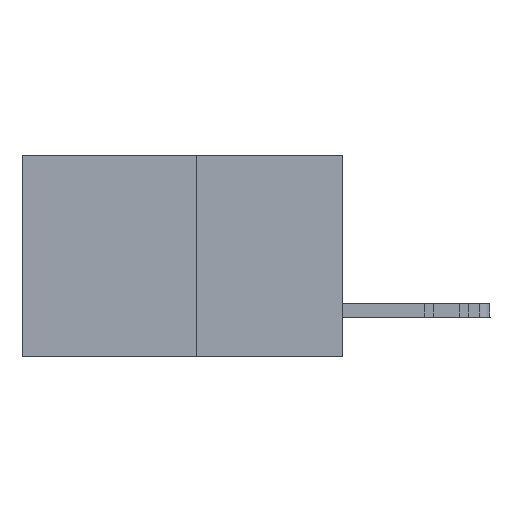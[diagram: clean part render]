
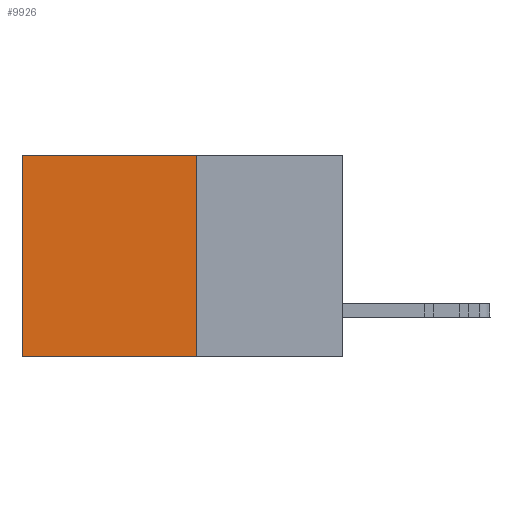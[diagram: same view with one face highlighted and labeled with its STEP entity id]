
A CAD part, left-side view. The second image highlights one B-rep face of the part: STEP entity #9926.
In plain terms, the highlighted planar face has unit normal (-1, 0, 0).
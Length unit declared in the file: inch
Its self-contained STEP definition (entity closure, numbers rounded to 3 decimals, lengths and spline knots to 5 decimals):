
#235 = DIRECTION ( 'NONE',  ( 0., 0., -1. ) ) ;
#756 = FACE_OUTER_BOUND ( 'NONE', #23919, .T. ) ;
#854 = ORIENTED_EDGE ( 'NONE', *, *, #23506, .F. ) ;
#917 = PLANE ( 'NONE',  #30844 ) ;
#5242 = VERTEX_POINT ( 'NONE', #9584 ) ;
#5549 = CARTESIAN_POINT ( 'NONE',  ( 0.277, 0.27, -0.37 ) ) ;
#5581 = DIRECTION ( 'NONE',  ( 0., 0., -1. ) ) ;
#5747 = CARTESIAN_POINT ( 'NONE',  ( 0.277, 0.27, -0.37 ) ) ;
#5979 = VERTEX_POINT ( 'NONE', #6456 ) ;
#6456 = CARTESIAN_POINT ( 'NONE',  ( 0.277, 0.27, 0. ) ) ;
#6889 = VECTOR ( 'NONE', #235, 39.37008 ) ;
#7749 = DIRECTION ( 'NONE',  ( 0., 1., 0. ) ) ;
#8254 = CARTESIAN_POINT ( 'NONE',  ( 0.277, 0.59, -0.37 ) ) ;
#9418 = CARTESIAN_POINT ( 'NONE',  ( 0.277, 0.59, 0. ) ) ;
#9584 = CARTESIAN_POINT ( 'NONE',  ( 0.277, 0.27, -0.37 ) ) ;
#9926 = ADVANCED_FACE ( 'NONE', ( #756 ), #917, .F. ) ;
#10907 = DIRECTION ( 'NONE',  ( 1., 0., 0. ) ) ;
#11306 = VECTOR ( 'NONE', #5581, 39.37008 ) ;
#12882 = CARTESIAN_POINT ( 'NONE',  ( 0.277, 0.59, -0.37 ) ) ;
#13426 = VECTOR ( 'NONE', #7749, 39.37008 ) ;
#14431 = EDGE_CURVE ( 'NONE', #5979, #14837, #25428, .T. ) ;
#14583 = EDGE_CURVE ( 'NONE', #14837, #31680, #20598, .T. ) ;
#14837 = VERTEX_POINT ( 'NONE', #9418 ) ;
#16862 = VECTOR ( 'NONE', #27567, 39.37008 ) ;
#17900 = LINE ( 'NONE', #5549, #6889 ) ;
#20426 = DIRECTION ( 'NONE',  ( 0., 0., -1. ) ) ;
#20598 = LINE ( 'NONE', #8254, #11306 ) ;
#21332 = EDGE_CURVE ( 'NONE', #5242, #31680, #32564, .T. ) ;
#23506 = EDGE_CURVE ( 'NONE', #5979, #5242, #17900, .T. ) ;
#23919 = EDGE_LOOP ( 'NONE', ( #27350, #31478, #854, #24360 ) ) ;
#24360 = ORIENTED_EDGE ( 'NONE', *, *, #14431, .T. ) ;
#25428 = LINE ( 'NONE', #30601, #13426 ) ;
#27350 = ORIENTED_EDGE ( 'NONE', *, *, #14583, .T. ) ;
#27567 = DIRECTION ( 'NONE',  ( 0., 1., 0. ) ) ;
#30065 = CARTESIAN_POINT ( 'NONE',  ( 0.277, 0.27, -0.37 ) ) ;
#30601 = CARTESIAN_POINT ( 'NONE',  ( 0.277, 0.27, 0. ) ) ;
#30844 = AXIS2_PLACEMENT_3D ( 'NONE', #5747, #10907, #20426 ) ;
#31478 = ORIENTED_EDGE ( 'NONE', *, *, #21332, .F. ) ;
#31680 = VERTEX_POINT ( 'NONE', #12882 ) ;
#32564 = LINE ( 'NONE', #30065, #16862 ) ;
